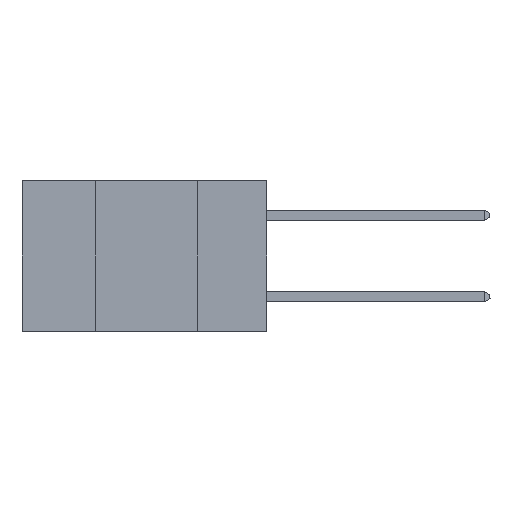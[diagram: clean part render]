
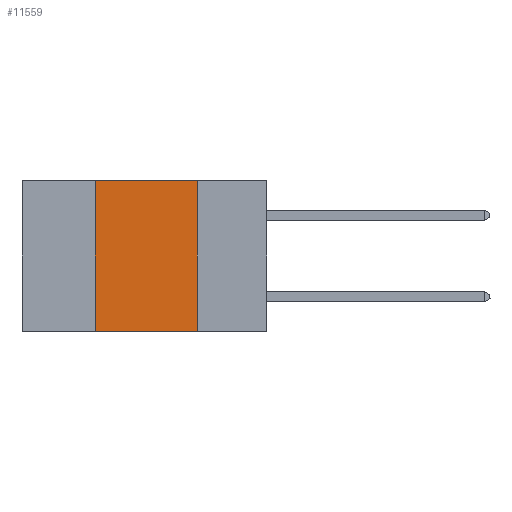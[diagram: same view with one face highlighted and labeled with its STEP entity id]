
A CAD part, left-side view. The second image highlights one B-rep face of the part: STEP entity #11559.
In plain terms, the highlighted planar face has unit normal (-1, 0, 0).
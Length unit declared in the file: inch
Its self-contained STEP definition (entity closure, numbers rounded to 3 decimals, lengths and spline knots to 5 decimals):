
#280 = VERTEX_POINT ( 'NONE', #18891 ) ;
#823 = EDGE_CURVE ( 'NONE', #280, #11296, #6842, .T. ) ;
#1211 = DIRECTION ( 'NONE',  ( 0., 0., -1. ) ) ;
#1722 = DIRECTION ( 'NONE',  ( 0., -1., 0. ) ) ;
#2477 = CARTESIAN_POINT ( 'NONE',  ( 0., 0.17, -0.37 ) ) ;
#3166 = FACE_OUTER_BOUND ( 'NONE', #16850, .T. ) ;
#4081 = CARTESIAN_POINT ( 'NONE',  ( 0., 0.17, 0. ) ) ;
#5057 = ORIENTED_EDGE ( 'NONE', *, *, #23742, .F. ) ;
#5682 = ORIENTED_EDGE ( 'NONE', *, *, #10201, .F. ) ;
#6842 = LINE ( 'NONE', #24959, #22208 ) ;
#7011 = DIRECTION ( 'NONE',  ( 0., 0., 1. ) ) ;
#7186 = LINE ( 'NONE', #12850, #15959 ) ;
#7264 = ORIENTED_EDGE ( 'NONE', *, *, #15233, .T. ) ;
#10201 = EDGE_CURVE ( 'NONE', #23996, #23062, #10915, .T. ) ;
#10867 = DIRECTION ( 'NONE',  ( 0., -1., 0. ) ) ;
#10915 = LINE ( 'NONE', #11258, #11524 ) ;
#11258 = CARTESIAN_POINT ( 'NONE',  ( 0., 0.17, 0. ) ) ;
#11296 = VERTEX_POINT ( 'NONE', #16184 ) ;
#11524 = VECTOR ( 'NONE', #13104, 39.37008 ) ;
#11559 = ADVANCED_FACE ( 'NONE', ( #3166 ), #23173, .F. ) ;
#11776 = AXIS2_PLACEMENT_3D ( 'NONE', #25125, #21215, #1211 ) ;
#11952 = ORIENTED_EDGE ( 'NONE', *, *, #823, .F. ) ;
#12850 = CARTESIAN_POINT ( 'NONE',  ( 0., 0.6, 0. ) ) ;
#13104 = DIRECTION ( 'NONE',  ( 0., 0., -1. ) ) ;
#13727 = CARTESIAN_POINT ( 'NONE',  ( 0., 0.6, -0.37 ) ) ;
#15233 = EDGE_CURVE ( 'NONE', #280, #23062, #22748, .T. ) ;
#15959 = VECTOR ( 'NONE', #10867, 39.37008 ) ;
#16184 = CARTESIAN_POINT ( 'NONE',  ( 0., 0.42, 0. ) ) ;
#16850 = EDGE_LOOP ( 'NONE', ( #5682, #5057, #11952, #7264 ) ) ;
#17730 = VECTOR ( 'NONE', #1722, 39.37008 ) ;
#18891 = CARTESIAN_POINT ( 'NONE',  ( 0., 0.42, -0.37 ) ) ;
#21215 = DIRECTION ( 'NONE',  ( 1., 0., 0. ) ) ;
#22208 = VECTOR ( 'NONE', #7011, 39.37008 ) ;
#22748 = LINE ( 'NONE', #13727, #17730 ) ;
#23062 = VERTEX_POINT ( 'NONE', #2477 ) ;
#23173 = PLANE ( 'NONE',  #11776 ) ;
#23742 = EDGE_CURVE ( 'NONE', #11296, #23996, #7186, .T. ) ;
#23996 = VERTEX_POINT ( 'NONE', #4081 ) ;
#24959 = CARTESIAN_POINT ( 'NONE',  ( 0., 0.42, 0. ) ) ;
#25125 = CARTESIAN_POINT ( 'NONE',  ( 0., 0.6, 0. ) ) ;
